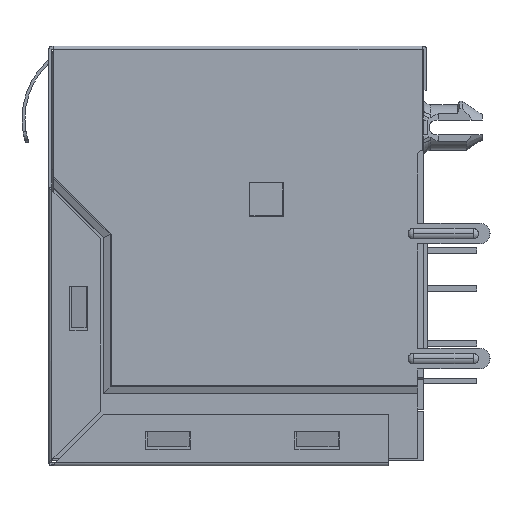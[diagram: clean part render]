
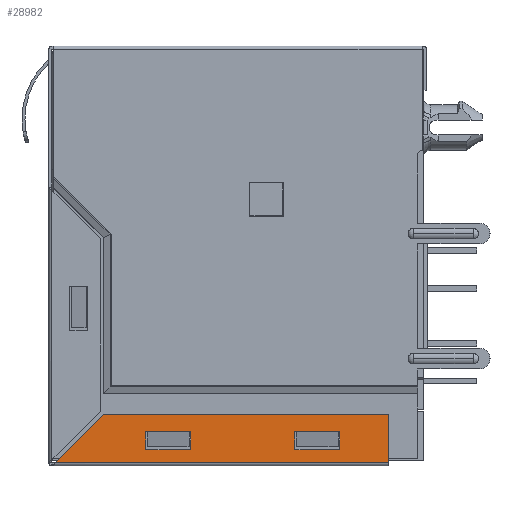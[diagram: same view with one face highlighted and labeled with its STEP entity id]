
A CAD part, left-side view. The second image highlights one B-rep face of the part: STEP entity #28982.
In plain terms, the highlighted planar face has unit normal (-1, 0, 0).
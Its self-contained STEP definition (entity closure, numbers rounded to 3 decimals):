
#711 = VERTEX_POINT ( 'NONE', #37213 ) ;
#5253 = B_SPLINE_CURVE_WITH_KNOTS ( 'NONE', 1,
 ( #20350, #54903 ),
 .UNSPECIFIED., .F., .F.,
 ( 2, 2 ),
 ( 0., 1. ),
 .UNSPECIFIED. ) ;
#5611 = EDGE_CURVE ( 'NONE', #66050, #69067, #71279, .T. ) ;
#5689 = ORIENTED_EDGE ( 'NONE', *, *, #40179, .T. ) ;
#5772 = CARTESIAN_POINT ( 'NONE',  ( -31.88, 6.165, -26.78 ) ) ;
#6784 = CARTESIAN_POINT ( 'NONE',  ( -31.88, 12.693, -27.79 ) ) ;
#6868 = CARTESIAN_POINT ( 'NONE',  ( -31.88, 3.165, -25.58 ) ) ;
#7546 = EDGE_CURVE ( 'NONE', #69067, #19316, #52192, .T. ) ;
#7843 = CARTESIAN_POINT ( 'NONE',  ( -31.88, 1.055, -27.67 ) ) ;
#8931 = EDGE_CURVE ( 'NONE', #711, #39802, #46057, .T. ) ;
#9044 = CARTESIAN_POINT ( 'NONE',  ( -31.88, 6.165, -25.58 ) ) ;
#9121 = CARTESIAN_POINT ( 'NONE',  ( -31.88, -10.135, -27.67 ) ) ;
#9178 = VERTEX_POINT ( 'NONE', #28368 ) ;
#12174 = EDGE_LOOP ( 'NONE', ( #59557, #72823, #75924, #5689 ) ) ;
#12943 = VERTEX_POINT ( 'NONE', #50264 ) ;
#13061 = FACE_OUTER_BOUND ( 'NONE', #43241, .T. ) ;
#14306 = LINE ( 'NONE', #7843, #72333 ) ;
#14365 = ORIENTED_EDGE ( 'NONE', *, *, #75730, .T. ) ;
#17022 = ORIENTED_EDGE ( 'NONE', *, *, #38616, .F. ) ;
#17046 = CARTESIAN_POINT ( 'NONE',  ( -31.88, 12.245, -27.67 ) ) ;
#17636 = EDGE_CURVE ( 'NONE', #39802, #60837, #72549, .T. ) ;
#18175 = CARTESIAN_POINT ( 'NONE',  ( -31.88, -10.135, -24.43 ) ) ;
#19316 = VERTEX_POINT ( 'NONE', #9044 ) ;
#19581 = B_SPLINE_CURVE_WITH_KNOTS ( 'NONE', 1,
 ( #51811, #17046 ),
 .UNSPECIFIED., .F., .F.,
 ( 2, 2 ),
 ( 0., 1. ),
 .UNSPECIFIED. ) ;
#20350 = CARTESIAN_POINT ( 'NONE',  ( -31.88, -3.835, -25.58 ) ) ;
#21916 = CARTESIAN_POINT ( 'NONE',  ( -31.88, -6.835, -25.58 ) ) ;
#22491 = EDGE_CURVE ( 'NONE', #12943, #28298, #19581, .T. ) ;
#23279 = CARTESIAN_POINT ( 'NONE',  ( -31.88, 3.165, -26.78 ) ) ;
#24693 = ORIENTED_EDGE ( 'NONE', *, *, #71653, .T. ) ;
#25039 = DIRECTION ( 'NONE',  ( 0., -1., 0. ) ) ;
#25240 = ORIENTED_EDGE ( 'NONE', *, *, #27100, .T. ) ;
#26673 = CARTESIAN_POINT ( 'NONE',  ( -31.88, 3.165, -26.78 ) ) ;
#26682 = CARTESIAN_POINT ( 'NONE',  ( -31.88, -10.135, -27.67 ) ) ;
#27100 = EDGE_CURVE ( 'NONE', #67570, #711, #55288, .T. ) ;
#27920 = CARTESIAN_POINT ( 'NONE',  ( -31.88, 3.165, -25.58 ) ) ;
#28077 = CARTESIAN_POINT ( 'NONE',  ( -31.88, 6.165, -26.78 ) ) ;
#28298 = VERTEX_POINT ( 'NONE', #43242 ) ;
#28368 = CARTESIAN_POINT ( 'NONE',  ( -31.88, 3.165, -25.58 ) ) ;
#28794 = CARTESIAN_POINT ( 'NONE',  ( -31.88, -3.835, -26.78 ) ) ;
#28982 = ADVANCED_FACE ( 'NONE', ( #13061, #70198, #60093 ), #60127, .T. ) ;
#29320 = CARTESIAN_POINT ( 'NONE',  ( -31.88, -3.835, -25.58 ) ) ;
#29931 = ORIENTED_EDGE ( 'NONE', *, *, #40422, .T. ) ;
#30039 = CARTESIAN_POINT ( 'NONE',  ( -31.88, 3.165, -26.78 ) ) ;
#30929 = B_SPLINE_CURVE_WITH_KNOTS ( 'NONE', 1,
 ( #66288, #54155 ),
 .UNSPECIFIED., .F., .F.,
 ( 2, 2 ),
 ( 0., 1. ),
 .UNSPECIFIED. ) ;
#31477 = CARTESIAN_POINT ( 'NONE',  ( -31.88, -6.835, -26.78 ) ) ;
#37213 = CARTESIAN_POINT ( 'NONE',  ( -31.88, -6.835, -26.78 ) ) ;
#37596 = VERTEX_POINT ( 'NONE', #9121 ) ;
#38616 = EDGE_CURVE ( 'NONE', #71582, #37596, #65434, .T. ) ;
#39802 = VERTEX_POINT ( 'NONE', #41599 ) ;
#39882 = CARTESIAN_POINT ( 'NONE',  ( -31.88, 6.165, -26.78 ) ) ;
#40179 = EDGE_CURVE ( 'NONE', #19316, #9178, #50317, .T. ) ;
#40422 = EDGE_CURVE ( 'NONE', #71582, #12943, #30929, .T. ) ;
#41599 = CARTESIAN_POINT ( 'NONE',  ( -31.88, -3.835, -26.78 ) ) ;
#41758 = ORIENTED_EDGE ( 'NONE', *, *, #17636, .T. ) ;
#43241 = EDGE_LOOP ( 'NONE', ( #17022, #29931, #46205, #24693 ) ) ;
#43242 = CARTESIAN_POINT ( 'NONE',  ( -31.88, 12.245, -27.67 ) ) ;
#43665 = B_SPLINE_CURVE_WITH_KNOTS ( 'NONE', 1,
 ( #6868, #30039 ),
 .UNSPECIFIED., .F., .F.,
 ( 2, 2 ),
 ( 0., 1. ),
 .UNSPECIFIED. ) ;
#46057 = B_SPLINE_CURVE_WITH_KNOTS ( 'NONE', 1,
 ( #31477, #61167 ),
 .UNSPECIFIED., .F., .F.,
 ( 2, 2 ),
 ( 0., 1. ),
 .UNSPECIFIED. ) ;
#46205 = ORIENTED_EDGE ( 'NONE', *, *, #22491, .T. ) ;
#47607 = EDGE_LOOP ( 'NONE', ( #25240, #50353, #41758, #14365 ) ) ;
#48780 = EDGE_CURVE ( 'NONE', #9178, #66050, #43665, .T. ) ;
#50264 = CARTESIAN_POINT ( 'NONE',  ( -31.88, 9.005, -24.43 ) ) ;
#50317 = B_SPLINE_CURVE_WITH_KNOTS ( 'NONE', 1,
 ( #57567, #27920 ),
 .UNSPECIFIED., .F., .F.,
 ( 2, 2 ),
 ( 0., 1. ),
 .UNSPECIFIED. ) ;
#50353 = ORIENTED_EDGE ( 'NONE', *, *, #8931, .T. ) ;
#50649 = CARTESIAN_POINT ( 'NONE',  ( -31.88, -10.135, -24.43 ) ) ;
#51811 = CARTESIAN_POINT ( 'NONE',  ( -31.88, 9.005, -24.43 ) ) ;
#52192 = B_SPLINE_CURVE_WITH_KNOTS ( 'NONE', 1,
 ( #39882, #74708 ),
 .UNSPECIFIED., .F., .F.,
 ( 2, 2 ),
 ( 0., 1. ),
 .UNSPECIFIED. ) ;
#52586 = CARTESIAN_POINT ( 'NONE',  ( -31.88, -3.835, -25.58 ) ) ;
#54155 = CARTESIAN_POINT ( 'NONE',  ( -31.88, 9.005, -24.43 ) ) ;
#54903 = CARTESIAN_POINT ( 'NONE',  ( -31.88, -6.835, -25.58 ) ) ;
#55288 = B_SPLINE_CURVE_WITH_KNOTS ( 'NONE', 1,
 ( #67175, #60759 ),
 .UNSPECIFIED., .F., .F.,
 ( 2, 2 ),
 ( 0., 1. ),
 .UNSPECIFIED. ) ;
#57567 = CARTESIAN_POINT ( 'NONE',  ( -31.88, 6.165, -25.58 ) ) ;
#59557 = ORIENTED_EDGE ( 'NONE', *, *, #48780, .T. ) ;
#59868 = DIRECTION ( 'NONE',  ( -1., 0., 0. ) ) ;
#60093 = FACE_BOUND ( 'NONE', #12174, .T. ) ;
#60127 = PLANE ( 'NONE',  #68940 ) ;
#60759 = CARTESIAN_POINT ( 'NONE',  ( -31.88, -6.835, -26.78 ) ) ;
#60837 = VERTEX_POINT ( 'NONE', #52586 ) ;
#61167 = CARTESIAN_POINT ( 'NONE',  ( -31.88, -3.835, -26.78 ) ) ;
#65434 = B_SPLINE_CURVE_WITH_KNOTS ( 'NONE', 1,
 ( #50649, #26682 ),
 .UNSPECIFIED., .F., .F.,
 ( 2, 2 ),
 ( 0., 1. ),
 .UNSPECIFIED. ) ;
#66050 = VERTEX_POINT ( 'NONE', #26673 ) ;
#66116 = DIRECTION ( 'NONE',  ( 0., -1., 0. ) ) ;
#66288 = CARTESIAN_POINT ( 'NONE',  ( -31.88, -10.135, -24.43 ) ) ;
#67175 = CARTESIAN_POINT ( 'NONE',  ( -31.88, -6.835, -25.58 ) ) ;
#67570 = VERTEX_POINT ( 'NONE', #21916 ) ;
#68940 = AXIS2_PLACEMENT_3D ( 'NONE', #6784, #59868, #25039 ) ;
#69067 = VERTEX_POINT ( 'NONE', #28077 ) ;
#70198 = FACE_BOUND ( 'NONE', #47607, .T. ) ;
#71279 = B_SPLINE_CURVE_WITH_KNOTS ( 'NONE', 1,
 ( #23279, #5772 ),
 .UNSPECIFIED., .F., .F.,
 ( 2, 2 ),
 ( 0., 1. ),
 .UNSPECIFIED. ) ;
#71582 = VERTEX_POINT ( 'NONE', #18175 ) ;
#71653 = EDGE_CURVE ( 'NONE', #28298, #37596, #14306, .T. ) ;
#72333 = VECTOR ( 'NONE', #66116, 1000. ) ;
#72549 = B_SPLINE_CURVE_WITH_KNOTS ( 'NONE', 1,
 ( #28794, #29320 ),
 .UNSPECIFIED., .F., .F.,
 ( 2, 2 ),
 ( 0., 1. ),
 .UNSPECIFIED. ) ;
#72823 = ORIENTED_EDGE ( 'NONE', *, *, #5611, .T. ) ;
#74708 = CARTESIAN_POINT ( 'NONE',  ( -31.88, 6.165, -25.58 ) ) ;
#75730 = EDGE_CURVE ( 'NONE', #60837, #67570, #5253, .T. ) ;
#75924 = ORIENTED_EDGE ( 'NONE', *, *, #7546, .T. ) ;
